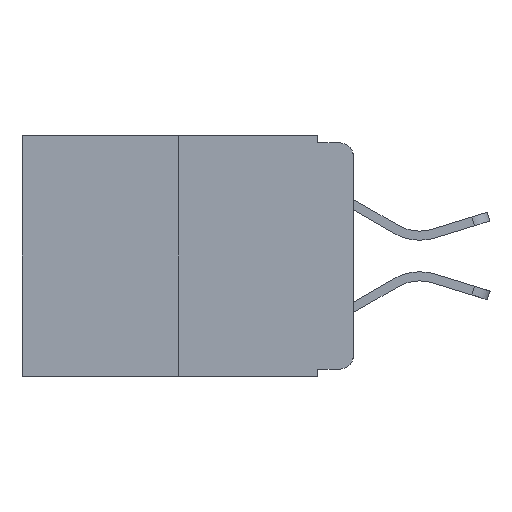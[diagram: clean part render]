
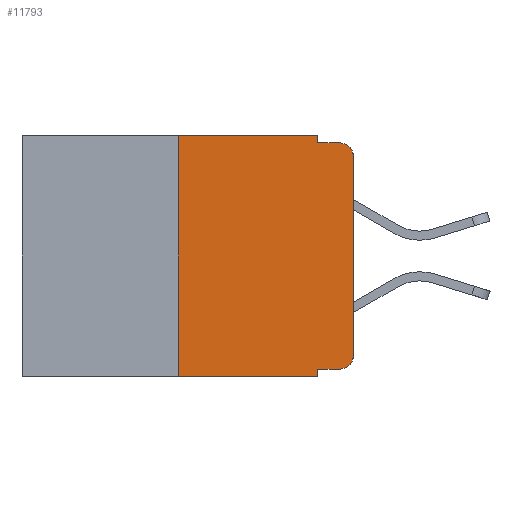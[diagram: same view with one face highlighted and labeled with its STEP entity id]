
A CAD part, left-side view. The second image highlights one B-rep face of the part: STEP entity #11793.
In plain terms, the highlighted planar face has unit normal (-1, 0, 0).
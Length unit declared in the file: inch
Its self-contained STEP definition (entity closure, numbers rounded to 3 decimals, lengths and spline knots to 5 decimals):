
#286 = ORIENTED_EDGE ( 'NONE', *, *, #10634, .T. ) ;
#853 = DIRECTION ( 'NONE',  ( 0., 0., -1. ) ) ;
#954 = VERTEX_POINT ( 'NONE', #12323 ) ;
#1170 = VECTOR ( 'NONE', #10041, 39.37008 ) ;
#1176 = VECTOR ( 'NONE', #853, 39.37008 ) ;
#1273 = LINE ( 'NONE', #4571, #5611 ) ;
#1884 = DIRECTION ( 'NONE',  ( 0., 0., -1. ) ) ;
#1903 = LINE ( 'NONE', #11627, #1176 ) ;
#2028 = CARTESIAN_POINT ( 'NONE',  ( 0., 0.25, -0.343 ) ) ;
#2507 = LINE ( 'NONE', #8215, #7233 ) ;
#2766 = LINE ( 'NONE', #3394, #5594 ) ;
#2987 = LINE ( 'NONE', #15148, #11437 ) ;
#3230 = FACE_OUTER_BOUND ( 'NONE', #12421, .T. ) ;
#3258 = CIRCLE ( 'NONE', #7361, 0.02 ) ;
#3288 = LINE ( 'NONE', #4420, #9345 ) ;
#3394 = CARTESIAN_POINT ( 'NONE',  ( 0., 0.473, 0. ) ) ;
#3617 = EDGE_CURVE ( 'NONE', #8042, #12233, #12338, .T. ) ;
#4157 = ORIENTED_EDGE ( 'NONE', *, *, #10665, .T. ) ;
#4258 = CARTESIAN_POINT ( 'NONE',  ( 0., 0.051, -0.333 ) ) ;
#4357 = DIRECTION ( 'NONE',  ( 0., -1., 0. ) ) ;
#4366 = EDGE_CURVE ( 'NONE', #954, #7743, #12688, .T. ) ;
#4420 = CARTESIAN_POINT ( 'NONE',  ( 0., 0.051, -0.01 ) ) ;
#4571 = CARTESIAN_POINT ( 'NONE',  ( 0., 0.473, -0.343 ) ) ;
#4594 = ORIENTED_EDGE ( 'NONE', *, *, #14301, .T. ) ;
#4617 = DIRECTION ( 'NONE',  ( 0., -1., 0. ) ) ;
#4815 = CARTESIAN_POINT ( 'NONE',  ( 0., 0.051, -0.343 ) ) ;
#5338 = EDGE_CURVE ( 'NONE', #14879, #954, #2987, .T. ) ;
#5566 = AXIS2_PLACEMENT_3D ( 'NONE', #10390, #12905, #8179 ) ;
#5594 = VECTOR ( 'NONE', #4617, 39.37008 ) ;
#5611 = VECTOR ( 'NONE', #9339, 39.37008 ) ;
#5785 = DIRECTION ( 'NONE',  ( -1., 0., 0. ) ) ;
#6406 = VERTEX_POINT ( 'NONE', #4258 ) ;
#6820 = DIRECTION ( 'NONE',  ( 0., 0., -1. ) ) ;
#6852 = ORIENTED_EDGE ( 'NONE', *, *, #9916, .F. ) ;
#6899 = EDGE_CURVE ( 'NONE', #6406, #11348, #1903, .T. ) ;
#7233 = VECTOR ( 'NONE', #15522, 39.37008 ) ;
#7361 = AXIS2_PLACEMENT_3D ( 'NONE', #14093, #5785, #6820 ) ;
#7372 = ORIENTED_EDGE ( 'NONE', *, *, #5338, .T. ) ;
#7644 = ORIENTED_EDGE ( 'NONE', *, *, #4366, .T. ) ;
#7743 = VERTEX_POINT ( 'NONE', #8298 ) ;
#7812 = CARTESIAN_POINT ( 'NONE',  ( 0., 0.051, 0. ) ) ;
#8042 = VERTEX_POINT ( 'NONE', #7812 ) ;
#8125 = PLANE ( 'NONE',  #5566 ) ;
#8152 = DIRECTION ( 'NONE',  ( 0., 0., 1. ) ) ;
#8179 = DIRECTION ( 'NONE',  ( 0., 0., -1. ) ) ;
#8215 = CARTESIAN_POINT ( 'NONE',  ( 0., 0.051, -0.333 ) ) ;
#8298 = CARTESIAN_POINT ( 'NONE',  ( 0., 0.02, -0.01 ) ) ;
#8695 = CARTESIAN_POINT ( 'NONE',  ( 0., 0.051, -0.01 ) ) ;
#8826 = EDGE_CURVE ( 'NONE', #10461, #8042, #2766, .T. ) ;
#9158 = VERTEX_POINT ( 'NONE', #9855 ) ;
#9278 = ORIENTED_EDGE ( 'NONE', *, *, #3617, .F. ) ;
#9339 = DIRECTION ( 'NONE',  ( 0., -1., 0. ) ) ;
#9345 = VECTOR ( 'NONE', #4357, 39.37008 ) ;
#9587 = DIRECTION ( 'NONE',  ( 0., 0., 1. ) ) ;
#9608 = LINE ( 'NONE', #15636, #15562 ) ;
#9855 = CARTESIAN_POINT ( 'NONE',  ( 0., 0.02, -0.333 ) ) ;
#9916 = EDGE_CURVE ( 'NONE', #12233, #7743, #3288, .T. ) ;
#10041 = DIRECTION ( 'NONE',  ( 0., 0., -1. ) ) ;
#10390 = CARTESIAN_POINT ( 'NONE',  ( 0., 0.473, 0. ) ) ;
#10461 = VERTEX_POINT ( 'NONE', #15273 ) ;
#10594 = CARTESIAN_POINT ( 'NONE',  ( 0., 0., -0.313 ) ) ;
#10634 = EDGE_CURVE ( 'NONE', #6406, #9158, #2507, .T. ) ;
#10665 = EDGE_CURVE ( 'NONE', #9158, #14879, #3258, .T. ) ;
#10726 = VERTEX_POINT ( 'NONE', #2028 ) ;
#10834 = ORIENTED_EDGE ( 'NONE', *, *, #8826, .F. ) ;
#11071 = AXIS2_PLACEMENT_3D ( 'NONE', #11481, #11685, #1884 ) ;
#11348 = VERTEX_POINT ( 'NONE', #4815 ) ;
#11437 = VECTOR ( 'NONE', #8152, 39.37008 ) ;
#11481 = CARTESIAN_POINT ( 'NONE',  ( 0., 0.02, -0.03 ) ) ;
#11627 = CARTESIAN_POINT ( 'NONE',  ( 0., 0.051, 0. ) ) ;
#11685 = DIRECTION ( 'NONE',  ( -1., 0., 0. ) ) ;
#11793 = ADVANCED_FACE ( 'NONE', ( #3230 ), #8125, .F. ) ;
#12233 = VERTEX_POINT ( 'NONE', #8695 ) ;
#12307 = ORIENTED_EDGE ( 'NONE', *, *, #13201, .F. ) ;
#12323 = CARTESIAN_POINT ( 'NONE',  ( 0., 0., -0.03 ) ) ;
#12338 = LINE ( 'NONE', #12464, #1170 ) ;
#12421 = EDGE_LOOP ( 'NONE', ( #7372, #7644, #6852, #9278, #10834, #12307, #4594, #15394, #286, #4157 ) ) ;
#12464 = CARTESIAN_POINT ( 'NONE',  ( 0., 0.051, 0. ) ) ;
#12688 = CIRCLE ( 'NONE', #11071, 0.02 ) ;
#12905 = DIRECTION ( 'NONE',  ( 1., 0., 0. ) ) ;
#13201 = EDGE_CURVE ( 'NONE', #10726, #10461, #9608, .T. ) ;
#14093 = CARTESIAN_POINT ( 'NONE',  ( 0., 0.02, -0.313 ) ) ;
#14301 = EDGE_CURVE ( 'NONE', #10726, #11348, #1273, .T. ) ;
#14879 = VERTEX_POINT ( 'NONE', #10594 ) ;
#15148 = CARTESIAN_POINT ( 'NONE',  ( 0., 0., 0. ) ) ;
#15273 = CARTESIAN_POINT ( 'NONE',  ( 0., 0.25, 0. ) ) ;
#15394 = ORIENTED_EDGE ( 'NONE', *, *, #6899, .F. ) ;
#15522 = DIRECTION ( 'NONE',  ( 0., -1., 0. ) ) ;
#15562 = VECTOR ( 'NONE', #9587, 39.37008 ) ;
#15636 = CARTESIAN_POINT ( 'NONE',  ( 0., 0.25, 0. ) ) ;
